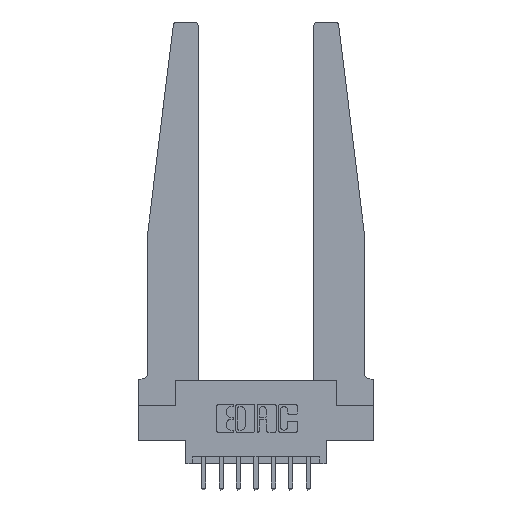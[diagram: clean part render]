
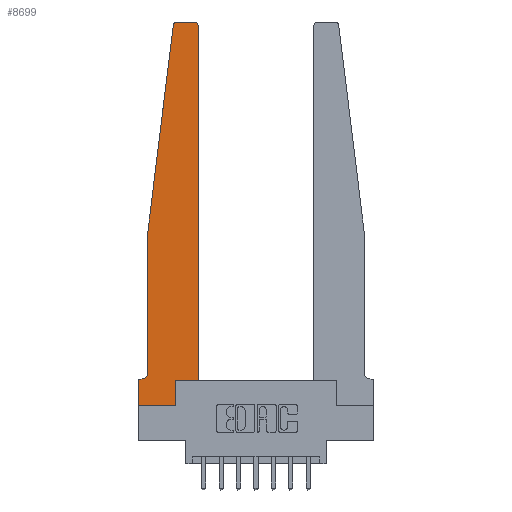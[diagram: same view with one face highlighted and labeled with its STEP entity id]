
A CAD part, top view. The second image highlights one B-rep face of the part: STEP entity #8699.
In plain terms, the highlighted planar face has unit normal (0, 0, 1).
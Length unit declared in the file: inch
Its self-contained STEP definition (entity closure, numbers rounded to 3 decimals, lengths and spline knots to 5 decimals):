
#54 = VERTEX_POINT ( 'NONE', #10907 ) ;
#223 = CARTESIAN_POINT ( 'NONE',  ( 0., 0.1875, 0.37 ) ) ;
#761 = CARTESIAN_POINT ( 'NONE',  ( 0.065, 1.25, 0.37 ) ) ;
#771 = VECTOR ( 'NONE', #1993, 39.37008 ) ;
#1624 = ORIENTED_EDGE ( 'NONE', *, *, #8200, .T. ) ;
#1668 = CARTESIAN_POINT ( 'NONE',  ( 0.065, 1.25, 0.37 ) ) ;
#1716 = PLANE ( 'NONE',  #2866 ) ;
#1759 = LINE ( 'NONE', #5227, #1937 ) ;
#1845 = ORIENTED_EDGE ( 'NONE', *, *, #4618, .T. ) ;
#1937 = VECTOR ( 'NONE', #5050, 39.37008 ) ;
#1957 = DIRECTION ( 'NONE',  ( -0.122, -0.992, 0. ) ) ;
#1993 = DIRECTION ( 'NONE',  ( -1., 0., 0. ) ) ;
#1995 = ORIENTED_EDGE ( 'NONE', *, *, #10741, .T. ) ;
#2034 = ORIENTED_EDGE ( 'NONE', *, *, #2810, .T. ) ;
#2073 = CARTESIAN_POINT ( 'NONE',  ( 0.015, 0.2375, 0.37 ) ) ;
#2336 = AXIS2_PLACEMENT_3D ( 'NONE', #2073, #9967, #3213 ) ;
#2440 = ORIENTED_EDGE ( 'NONE', *, *, #11759, .T. ) ;
#2455 = VECTOR ( 'NONE', #9775, 39.37008 ) ;
#2543 = CARTESIAN_POINT ( 'NONE',  ( 0.395, 2.75, 0.37 ) ) ;
#2588 = ORIENTED_EDGE ( 'NONE', *, *, #5335, .T. ) ;
#2629 = VERTEX_POINT ( 'NONE', #8746 ) ;
#2742 = ORIENTED_EDGE ( 'NONE', *, *, #11832, .T. ) ;
#2810 = EDGE_CURVE ( 'NONE', #12329, #5285, #9220, .T. ) ;
#2854 = DIRECTION ( 'NONE',  ( 1., 0., 0. ) ) ;
#2866 = AXIS2_PLACEMENT_3D ( 'NONE', #12795, #9636, #2854 ) ;
#2974 = LINE ( 'NONE', #10139, #2455 ) ;
#3049 = CARTESIAN_POINT ( 'NONE',  ( 0.425, 0.18, 0.37 ) ) ;
#3053 = VERTEX_POINT ( 'NONE', #3425 ) ;
#3094 = ORIENTED_EDGE ( 'NONE', *, *, #3885, .T. ) ;
#3213 = DIRECTION ( 'NONE',  ( -1., 0., 0. ) ) ;
#3356 = ORIENTED_EDGE ( 'NONE', *, *, #3417, .T. ) ;
#3361 = VERTEX_POINT ( 'NONE', #13906 ) ;
#3417 = EDGE_CURVE ( 'NONE', #54, #14071, #5266, .T. ) ;
#3425 = CARTESIAN_POINT ( 'NONE',  ( 0.24675, 2.72367, 0.37 ) ) ;
#3585 = ORIENTED_EDGE ( 'NONE', *, *, #3989, .T. ) ;
#3666 = ORIENTED_EDGE ( 'NONE', *, *, #11249, .T. ) ;
#3765 = VERTEX_POINT ( 'NONE', #11654 ) ;
#3777 = ORIENTED_EDGE ( 'NONE', *, *, #7831, .T. ) ;
#3885 = EDGE_CURVE ( 'NONE', #3361, #54, #2974, .T. ) ;
#3989 = EDGE_CURVE ( 'NONE', #14071, #10120, #1759, .T. ) ;
#4161 = LINE ( 'NONE', #761, #7235 ) ;
#4169 = CARTESIAN_POINT ( 'NONE',  ( 0.2605, 0.18, 0.37 ) ) ;
#4618 = EDGE_CURVE ( 'NONE', #2629, #3053, #12966, .T. ) ;
#4643 = DIRECTION ( 'NONE',  ( 1., 0., 0. ) ) ;
#4749 = DIRECTION ( 'NONE',  ( 0., 0., 1. ) ) ;
#4796 = DIRECTION ( 'NONE',  ( 0., 0., 1. ) ) ;
#4903 = CARTESIAN_POINT ( 'NONE',  ( 0.27653, 2.72, 0.37 ) ) ;
#5050 = DIRECTION ( 'NONE',  ( 1., 0., 0. ) ) ;
#5061 = VECTOR ( 'NONE', #11010, 39.37008 ) ;
#5227 = CARTESIAN_POINT ( 'NONE',  ( 0.425, 0.18, 0.37 ) ) ;
#5266 = LINE ( 'NONE', #11152, #5061 ) ;
#5285 = VERTEX_POINT ( 'NONE', #12360 ) ;
#5335 = EDGE_CURVE ( 'NONE', #6820, #6006, #9232, .T. ) ;
#5582 = CARTESIAN_POINT ( 'NONE',  ( 0.425, 0.18, 0.37 ) ) ;
#5691 = DIRECTION ( 'NONE',  ( 0., -1., 0. ) ) ;
#5747 = CARTESIAN_POINT ( 'NONE',  ( 0.015, 0.1875, 0.37 ) ) ;
#6006 = VERTEX_POINT ( 'NONE', #223 ) ;
#6136 = CIRCLE ( 'NONE', #2336, 0.05 ) ;
#6682 = CARTESIAN_POINT ( 'NONE',  ( 0.065, 1.25, 0.37 ) ) ;
#6820 = VERTEX_POINT ( 'NONE', #5747 ) ;
#6835 = AXIS2_PLACEMENT_3D ( 'NONE', #11353, #4796, #12431 ) ;
#6863 = LINE ( 'NONE', #5582, #12261 ) ;
#6866 = DIRECTION ( 'NONE',  ( 0., -1., 0. ) ) ;
#7235 = VECTOR ( 'NONE', #1957, 39.37008 ) ;
#7831 = EDGE_CURVE ( 'NONE', #3765, #12711, #10025, .T. ) ;
#8078 = LINE ( 'NONE', #12187, #13980 ) ;
#8200 = EDGE_CURVE ( 'NONE', #12711, #2629, #9181, .T. ) ;
#8471 = FACE_OUTER_BOUND ( 'NONE', #9083, .T. ) ;
#8699 = ADVANCED_FACE ( 'NONE', ( #8471 ), #1716, .T. ) ;
#8746 = CARTESIAN_POINT ( 'NONE',  ( 0.27653, 2.75, 0.37 ) ) ;
#9083 = EDGE_LOOP ( 'NONE', ( #1624, #1845, #1995, #2034, #2440, #2588, #2742, #3094, #3356, #3585, #3666, #3777 ) ) ;
#9181 = LINE ( 'NONE', #9756, #771 ) ;
#9195 = VECTOR ( 'NONE', #6866, 39.37008 ) ;
#9203 = VECTOR ( 'NONE', #11392, 39.37008 ) ;
#9220 = LINE ( 'NONE', #6682, #9195 ) ;
#9232 = LINE ( 'NONE', #11425, #9203 ) ;
#9636 = DIRECTION ( 'NONE',  ( 0., 0., 1. ) ) ;
#9756 = CARTESIAN_POINT ( 'NONE',  ( 0.25, 2.75, 0.37 ) ) ;
#9775 = DIRECTION ( 'NONE',  ( 1., 0., 0. ) ) ;
#9909 = AXIS2_PLACEMENT_3D ( 'NONE', #4903, #4749, #4643 ) ;
#9967 = DIRECTION ( 'NONE',  ( 0., 0., -1. ) ) ;
#10025 = CIRCLE ( 'NONE', #6835, 0.03 ) ;
#10120 = VERTEX_POINT ( 'NONE', #3049 ) ;
#10139 = CARTESIAN_POINT ( 'NONE',  ( 0., 0., 0.37 ) ) ;
#10741 = EDGE_CURVE ( 'NONE', #3053, #12329, #4161, .T. ) ;
#10907 = CARTESIAN_POINT ( 'NONE',  ( 0.2605, 0., 0.37 ) ) ;
#11010 = DIRECTION ( 'NONE',  ( 0., 1., 0. ) ) ;
#11152 = CARTESIAN_POINT ( 'NONE',  ( 0.2605, 0.18, 0.37 ) ) ;
#11249 = EDGE_CURVE ( 'NONE', #10120, #3765, #6863, .T. ) ;
#11353 = CARTESIAN_POINT ( 'NONE',  ( 0.395, 2.72, 0.37 ) ) ;
#11392 = DIRECTION ( 'NONE',  ( -1., 0., 0. ) ) ;
#11425 = CARTESIAN_POINT ( 'NONE',  ( 0.065, 0.1875, 0.37 ) ) ;
#11654 = CARTESIAN_POINT ( 'NONE',  ( 0.425, 2.72, 0.37 ) ) ;
#11759 = EDGE_CURVE ( 'NONE', #5285, #6820, #6136, .T. ) ;
#11832 = EDGE_CURVE ( 'NONE', #6006, #3361, #8078, .T. ) ;
#12187 = CARTESIAN_POINT ( 'NONE',  ( 0., 0., 0.37 ) ) ;
#12261 = VECTOR ( 'NONE', #14102, 39.37008 ) ;
#12329 = VERTEX_POINT ( 'NONE', #1668 ) ;
#12360 = CARTESIAN_POINT ( 'NONE',  ( 0.065, 0.2375, 0.37 ) ) ;
#12431 = DIRECTION ( 'NONE',  ( 1., 0., 0. ) ) ;
#12711 = VERTEX_POINT ( 'NONE', #2543 ) ;
#12795 = CARTESIAN_POINT ( 'NONE',  ( 0., 0.1875, 0.37 ) ) ;
#12966 = CIRCLE ( 'NONE', #9909, 0.03 ) ;
#13906 = CARTESIAN_POINT ( 'NONE',  ( 0., 0., 0.37 ) ) ;
#13980 = VECTOR ( 'NONE', #5691, 39.37008 ) ;
#14071 = VERTEX_POINT ( 'NONE', #4169 ) ;
#14102 = DIRECTION ( 'NONE',  ( 0., 1., 0. ) ) ;
